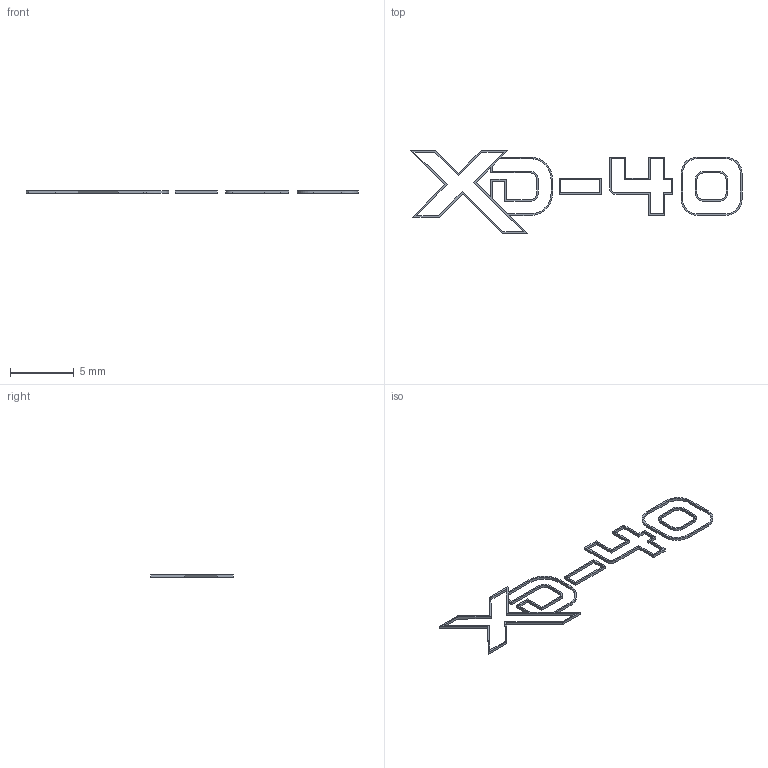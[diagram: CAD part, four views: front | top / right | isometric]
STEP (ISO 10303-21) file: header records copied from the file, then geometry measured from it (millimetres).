
FILE_DESCRIPTION (( 'STEP AP214' ), '1' );
FILE_NAME ('ENGRAVING FILL - XD-40.STEP', '2013-06-19T14:02:47', ( 'Asher' ), ( '' ), 'SwSTEP 2.0', 'SolidWorks 2013', '' );
FILE_SCHEMA (( 'AUTOMOTIVE_DESIGN' ));
Length unit declared in the file: millimetre
Products named in the file (1): ENGRAVING FILL - XD-40
Bounding box: 25.94 x 6.48 x 0.2 mm (x, y, z)
Volume: 2.9 mm3; surface area: 74.5 mm2
Topology: 5 solids, 5 shells, 136 faces, 378 edges, 252 vertices
Faces by surface type: plane 110, cylinder 26
Entity records: 4412 total; most frequent: CARTESIAN_POINT 767, ORIENTED_EDGE 756, DIRECTION 704, EDGE_CURVE 378, VECTOR 326, LINE 326, VERTEX_POINT 252, AXIS2_PLACEMENT_3D 189
